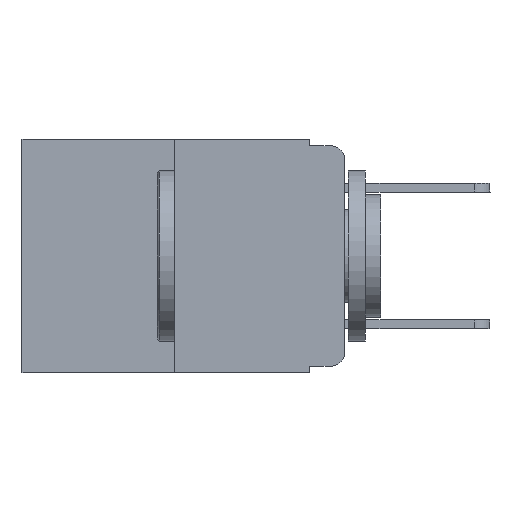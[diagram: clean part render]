
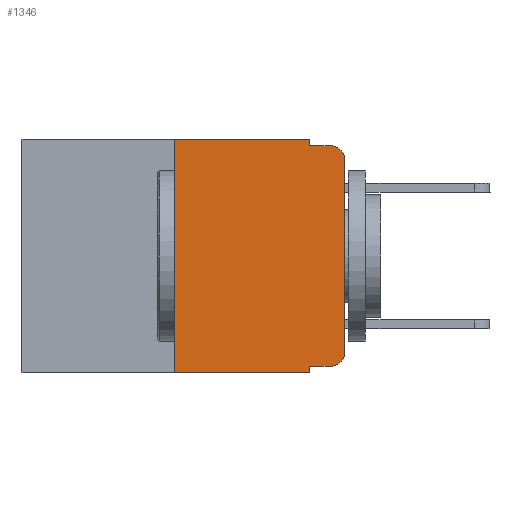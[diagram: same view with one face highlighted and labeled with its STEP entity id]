
A CAD part, left-side view. The second image highlights one B-rep face of the part: STEP entity #1346.
In plain terms, the highlighted planar face has unit normal (-1, 0, 0).
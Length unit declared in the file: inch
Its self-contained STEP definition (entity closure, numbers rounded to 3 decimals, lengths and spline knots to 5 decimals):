
#263 = EDGE_CURVE ( 'NONE', #4018, #1508, #873, .T. ) ;
#313 = LINE ( 'NONE', #7510, #2268 ) ;
#331 = CARTESIAN_POINT ( 'NONE',  ( 0., 0.02, -0.333 ) ) ;
#502 = DIRECTION ( 'NONE',  ( 0., 0., 1. ) ) ;
#545 = ORIENTED_EDGE ( 'NONE', *, *, #7688, .F. ) ;
#749 = VERTEX_POINT ( 'NONE', #6283 ) ;
#873 = LINE ( 'NONE', #9571, #8443 ) ;
#1175 = DIRECTION ( 'NONE',  ( 0., 0., -1. ) ) ;
#1346 = ADVANCED_FACE ( 'NONE', ( #9872 ), #6502, .F. ) ;
#1357 = VECTOR ( 'NONE', #1175, 39.37008 ) ;
#1400 = VERTEX_POINT ( 'NONE', #3865 ) ;
#1482 = AXIS2_PLACEMENT_3D ( 'NONE', #6628, #7538, #1666 ) ;
#1501 = VECTOR ( 'NONE', #502, 39.37008 ) ;
#1508 = VERTEX_POINT ( 'NONE', #331 ) ;
#1549 = CARTESIAN_POINT ( 'NONE',  ( 0., 0.473, 0. ) ) ;
#1666 = DIRECTION ( 'NONE',  ( 0., 0., -1. ) ) ;
#1786 = VERTEX_POINT ( 'NONE', #6516 ) ;
#2268 = VECTOR ( 'NONE', #5001, 39.37008 ) ;
#2314 = CARTESIAN_POINT ( 'NONE',  ( 0., 0.051, 0. ) ) ;
#2616 = ORIENTED_EDGE ( 'NONE', *, *, #10106, .T. ) ;
#2657 = LINE ( 'NONE', #4462, #9825 ) ;
#2857 = VECTOR ( 'NONE', #3305, 39.37008 ) ;
#2883 = CARTESIAN_POINT ( 'NONE',  ( 0., 0.25, 0. ) ) ;
#3084 = CARTESIAN_POINT ( 'NONE',  ( 0., 0.473, 0. ) ) ;
#3121 = VERTEX_POINT ( 'NONE', #7668 ) ;
#3135 = CARTESIAN_POINT ( 'NONE',  ( 0., 0.051, -0.343 ) ) ;
#3159 = DIRECTION ( 'NONE',  ( 0., 0., -1. ) ) ;
#3170 = AXIS2_PLACEMENT_3D ( 'NONE', #4922, #10734, #4956 ) ;
#3209 = CARTESIAN_POINT ( 'NONE',  ( 0., 0.051, -0.01 ) ) ;
#3305 = DIRECTION ( 'NONE',  ( 0., -1., 0. ) ) ;
#3439 = ORIENTED_EDGE ( 'NONE', *, *, #10034, .T. ) ;
#3552 = CARTESIAN_POINT ( 'NONE',  ( 0., 0.25, -0.343 ) ) ;
#3763 = LINE ( 'NONE', #1549, #2857 ) ;
#3865 = CARTESIAN_POINT ( 'NONE',  ( 0., 0.051, 0. ) ) ;
#3937 = DIRECTION ( 'NONE',  ( 0., 0., -1. ) ) ;
#4010 = CARTESIAN_POINT ( 'NONE',  ( 0., 0., -0.03 ) ) ;
#4018 = VERTEX_POINT ( 'NONE', #8896 ) ;
#4130 = ORIENTED_EDGE ( 'NONE', *, *, #6504, .T. ) ;
#4263 = EDGE_CURVE ( 'NONE', #3121, #1400, #3763, .T. ) ;
#4441 = LINE ( 'NONE', #3209, #6802 ) ;
#4462 = CARTESIAN_POINT ( 'NONE',  ( 0., 0., 0. ) ) ;
#4698 = VERTEX_POINT ( 'NONE', #7182 ) ;
#4922 = CARTESIAN_POINT ( 'NONE',  ( 0., 0.02, -0.313 ) ) ;
#4956 = DIRECTION ( 'NONE',  ( 0., 0., -1. ) ) ;
#5001 = DIRECTION ( 'NONE',  ( 0., -1., 0. ) ) ;
#5073 = VERTEX_POINT ( 'NONE', #4010 ) ;
#5198 = ORIENTED_EDGE ( 'NONE', *, *, #6223, .F. ) ;
#5568 = DIRECTION ( 'NONE',  ( 0., -1., 0. ) ) ;
#6003 = CIRCLE ( 'NONE', #1482, 0.02 ) ;
#6052 = VECTOR ( 'NONE', #3159, 39.37008 ) ;
#6223 = EDGE_CURVE ( 'NONE', #7216, #3121, #6328, .T. ) ;
#6283 = CARTESIAN_POINT ( 'NONE',  ( 0., 0.051, -0.01 ) ) ;
#6318 = ORIENTED_EDGE ( 'NONE', *, *, #4263, .F. ) ;
#6328 = LINE ( 'NONE', #2883, #1501 ) ;
#6463 = DIRECTION ( 'NONE',  ( 1., 0., 0. ) ) ;
#6502 = PLANE ( 'NONE',  #7699 ) ;
#6504 = EDGE_CURVE ( 'NONE', #7216, #6924, #313, .T. ) ;
#6516 = CARTESIAN_POINT ( 'NONE',  ( 0., 0., -0.313 ) ) ;
#6543 = ORIENTED_EDGE ( 'NONE', *, *, #7340, .F. ) ;
#6628 = CARTESIAN_POINT ( 'NONE',  ( 0., 0.02, -0.03 ) ) ;
#6802 = VECTOR ( 'NONE', #5568, 39.37008 ) ;
#6839 = DIRECTION ( 'NONE',  ( 0., 0., 1. ) ) ;
#6924 = VERTEX_POINT ( 'NONE', #3135 ) ;
#7182 = CARTESIAN_POINT ( 'NONE',  ( 0., 0.02, -0.01 ) ) ;
#7216 = VERTEX_POINT ( 'NONE', #3552 ) ;
#7334 = ORIENTED_EDGE ( 'NONE', *, *, #7832, .T. ) ;
#7340 = EDGE_CURVE ( 'NONE', #4018, #6924, #9709, .T. ) ;
#7510 = CARTESIAN_POINT ( 'NONE',  ( 0., 0.473, -0.343 ) ) ;
#7538 = DIRECTION ( 'NONE',  ( -1., 0., 0. ) ) ;
#7668 = CARTESIAN_POINT ( 'NONE',  ( 0., 0.25, 0. ) ) ;
#7688 = EDGE_CURVE ( 'NONE', #1400, #749, #10467, .T. ) ;
#7699 = AXIS2_PLACEMENT_3D ( 'NONE', #3084, #6463, #3937 ) ;
#7832 = EDGE_CURVE ( 'NONE', #1786, #5073, #2657, .T. ) ;
#7834 = CARTESIAN_POINT ( 'NONE',  ( 0., 0.051, 0. ) ) ;
#7840 = DIRECTION ( 'NONE',  ( 0., -1., 0. ) ) ;
#7998 = ORIENTED_EDGE ( 'NONE', *, *, #9973, .F. ) ;
#8443 = VECTOR ( 'NONE', #7840, 39.37008 ) ;
#8896 = CARTESIAN_POINT ( 'NONE',  ( 0., 0.051, -0.333 ) ) ;
#9119 = CIRCLE ( 'NONE', #3170, 0.02 ) ;
#9564 = ORIENTED_EDGE ( 'NONE', *, *, #263, .T. ) ;
#9571 = CARTESIAN_POINT ( 'NONE',  ( 0., 0.051, -0.333 ) ) ;
#9709 = LINE ( 'NONE', #7834, #1357 ) ;
#9825 = VECTOR ( 'NONE', #6839, 39.37008 ) ;
#9872 = FACE_OUTER_BOUND ( 'NONE', #10124, .T. ) ;
#9973 = EDGE_CURVE ( 'NONE', #749, #4698, #4441, .T. ) ;
#10034 = EDGE_CURVE ( 'NONE', #5073, #4698, #6003, .T. ) ;
#10106 = EDGE_CURVE ( 'NONE', #1508, #1786, #9119, .T. ) ;
#10124 = EDGE_LOOP ( 'NONE', ( #7334, #3439, #7998, #545, #6318, #5198, #4130, #6543, #9564, #2616 ) ) ;
#10467 = LINE ( 'NONE', #2314, #6052 ) ;
#10734 = DIRECTION ( 'NONE',  ( -1., 0., 0. ) ) ;
